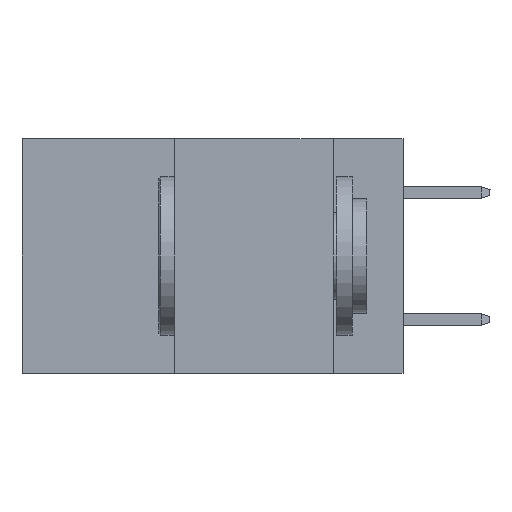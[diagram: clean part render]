
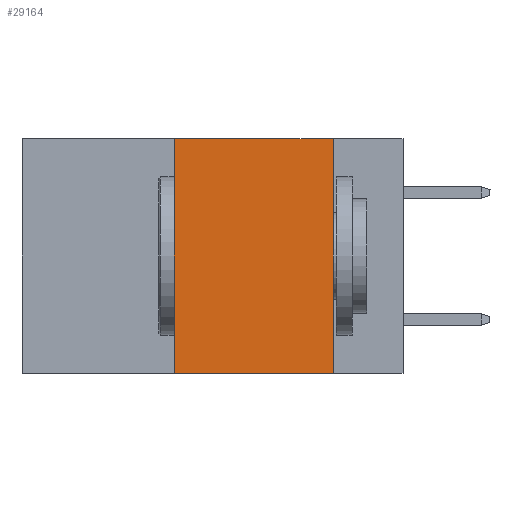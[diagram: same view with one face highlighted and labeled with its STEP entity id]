
A CAD part, left-side view. The second image highlights one B-rep face of the part: STEP entity #29164.
In plain terms, the highlighted planar face has unit normal (-1, 0, 0).
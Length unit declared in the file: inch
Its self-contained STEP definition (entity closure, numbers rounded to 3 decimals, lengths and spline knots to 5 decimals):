
#783 = VECTOR ( 'NONE', #19107, 39.37008 ) ;
#1170 = EDGE_CURVE ( 'NONE', #5301, #3601, #10725, .T. ) ;
#3433 = CARTESIAN_POINT ( 'NONE',  ( 0., 0.6, -0.37 ) ) ;
#3601 = VERTEX_POINT ( 'NONE', #17967 ) ;
#3967 = LINE ( 'NONE', #27021, #19112 ) ;
#5301 = VERTEX_POINT ( 'NONE', #31853 ) ;
#5426 = EDGE_CURVE ( 'NONE', #26357, #5301, #3967, .T. ) ;
#7834 = LINE ( 'NONE', #10610, #783 ) ;
#9156 = LINE ( 'NONE', #3433, #30268 ) ;
#9276 = FACE_OUTER_BOUND ( 'NONE', #28373, .T. ) ;
#10610 = CARTESIAN_POINT ( 'NONE',  ( 0., 0.11, 0. ) ) ;
#10725 = LINE ( 'NONE', #33253, #11200 ) ;
#11200 = VECTOR ( 'NONE', #28080, 39.37008 ) ;
#11501 = PLANE ( 'NONE',  #30037 ) ;
#15755 = VERTEX_POINT ( 'NONE', #22838 ) ;
#15931 = EDGE_CURVE ( 'NONE', #26357, #15755, #9156, .T. ) ;
#17429 = EDGE_CURVE ( 'NONE', #3601, #15755, #7834, .T. ) ;
#17967 = CARTESIAN_POINT ( 'NONE',  ( 0., 0.11, 0. ) ) ;
#19107 = DIRECTION ( 'NONE',  ( 0., 0., -1. ) ) ;
#19112 = VECTOR ( 'NONE', #29980, 39.37008 ) ;
#22648 = ORIENTED_EDGE ( 'NONE', *, *, #1170, .F. ) ;
#22838 = CARTESIAN_POINT ( 'NONE',  ( 0., 0.11, -0.37 ) ) ;
#23984 = CARTESIAN_POINT ( 'NONE',  ( 0., 0.36, -0.37 ) ) ;
#26357 = VERTEX_POINT ( 'NONE', #23984 ) ;
#27021 = CARTESIAN_POINT ( 'NONE',  ( 0., 0.36, 0. ) ) ;
#28080 = DIRECTION ( 'NONE',  ( 0., -1., 0. ) ) ;
#28373 = EDGE_LOOP ( 'NONE', ( #35207, #22648, #31535, #36152 ) ) ;
#28479 = CARTESIAN_POINT ( 'NONE',  ( 0., 0.6, 0. ) ) ;
#29164 = ADVANCED_FACE ( 'NONE', ( #9276 ), #11501, .F. ) ;
#29980 = DIRECTION ( 'NONE',  ( 0., 0., 1. ) ) ;
#30037 = AXIS2_PLACEMENT_3D ( 'NONE', #28479, #34568, #31439 ) ;
#30268 = VECTOR ( 'NONE', #32225, 39.37008 ) ;
#31439 = DIRECTION ( 'NONE',  ( 0., 0., -1. ) ) ;
#31535 = ORIENTED_EDGE ( 'NONE', *, *, #5426, .F. ) ;
#31853 = CARTESIAN_POINT ( 'NONE',  ( 0., 0.36, 0. ) ) ;
#32225 = DIRECTION ( 'NONE',  ( 0., -1., 0. ) ) ;
#33253 = CARTESIAN_POINT ( 'NONE',  ( 0., 0.6, 0. ) ) ;
#34568 = DIRECTION ( 'NONE',  ( 1., 0., 0. ) ) ;
#35207 = ORIENTED_EDGE ( 'NONE', *, *, #17429, .F. ) ;
#36152 = ORIENTED_EDGE ( 'NONE', *, *, #15931, .T. ) ;
